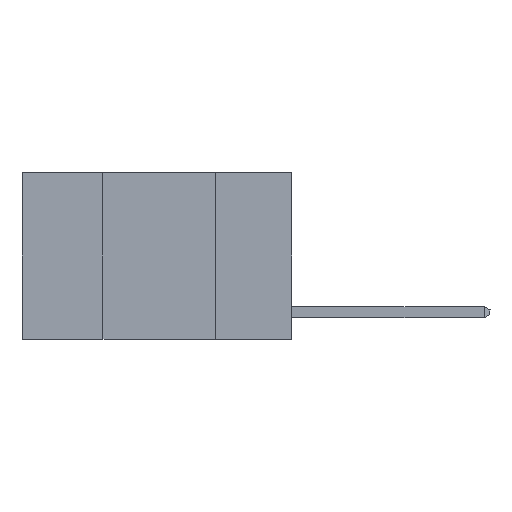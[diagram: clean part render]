
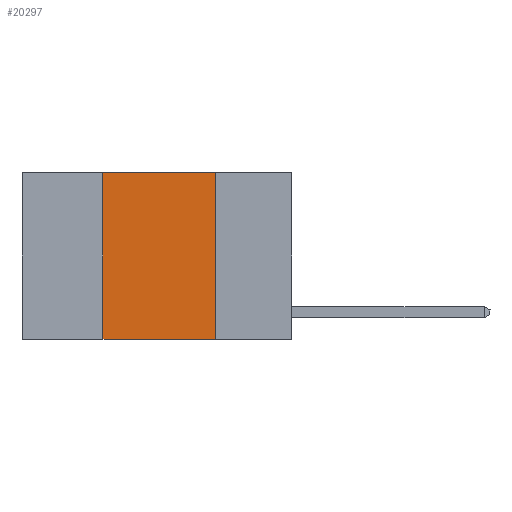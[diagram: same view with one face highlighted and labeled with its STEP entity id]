
A CAD part, left-side view. The second image highlights one B-rep face of the part: STEP entity #20297.
In plain terms, the highlighted planar face has unit normal (-1, 0, 0).
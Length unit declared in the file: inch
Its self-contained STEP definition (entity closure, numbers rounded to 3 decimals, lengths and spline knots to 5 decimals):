
#230 = VERTEX_POINT ( 'NONE', #10636 ) ;
#394 = DIRECTION ( 'NONE',  ( 0., -1., 0. ) ) ;
#1284 = ORIENTED_EDGE ( 'NONE', *, *, #28548, .F. ) ;
#4585 = LINE ( 'NONE', #11406, #22879 ) ;
#5337 = EDGE_CURVE ( 'NONE', #27834, #230, #9714, .T. ) ;
#9714 = LINE ( 'NONE', #11836, #29924 ) ;
#10095 = DIRECTION ( 'NONE',  ( 0., 0., -1. ) ) ;
#10636 = CARTESIAN_POINT ( 'NONE',  ( 0., 0.17, -0.37 ) ) ;
#11406 = CARTESIAN_POINT ( 'NONE',  ( 0., 0.42, 0. ) ) ;
#11836 = CARTESIAN_POINT ( 'NONE',  ( 0., 0.17, 0. ) ) ;
#11877 = CARTESIAN_POINT ( 'NONE',  ( 0., 0.17, 0. ) ) ;
#13815 = DIRECTION ( 'NONE',  ( 0., 0., -1. ) ) ;
#14064 = CARTESIAN_POINT ( 'NONE',  ( 0., 0.6, -0.37 ) ) ;
#15470 = AXIS2_PLACEMENT_3D ( 'NONE', #17219, #26232, #10095 ) ;
#17023 = ORIENTED_EDGE ( 'NONE', *, *, #5337, .F. ) ;
#17112 = ORIENTED_EDGE ( 'NONE', *, *, #17234, .T. ) ;
#17219 = CARTESIAN_POINT ( 'NONE',  ( 0., 0.6, 0. ) ) ;
#17224 = CARTESIAN_POINT ( 'NONE',  ( 0., 0.42, -0.37 ) ) ;
#17234 = EDGE_CURVE ( 'NONE', #21614, #230, #25637, .T. ) ;
#20297 = ADVANCED_FACE ( 'NONE', ( #23789 ), #28659, .F. ) ;
#20781 = VECTOR ( 'NONE', #394, 39.37008 ) ;
#21614 = VERTEX_POINT ( 'NONE', #17224 ) ;
#22252 = EDGE_CURVE ( 'NONE', #21614, #23963, #4585, .T. ) ;
#22475 = LINE ( 'NONE', #25357, #27210 ) ;
#22777 = DIRECTION ( 'NONE',  ( 0., -1., 0. ) ) ;
#22879 = VECTOR ( 'NONE', #25560, 39.37008 ) ;
#23789 = FACE_OUTER_BOUND ( 'NONE', #26074, .T. ) ;
#23963 = VERTEX_POINT ( 'NONE', #28694 ) ;
#25357 = CARTESIAN_POINT ( 'NONE',  ( 0., 0.6, 0. ) ) ;
#25560 = DIRECTION ( 'NONE',  ( 0., 0., 1. ) ) ;
#25637 = LINE ( 'NONE', #14064, #20781 ) ;
#26074 = EDGE_LOOP ( 'NONE', ( #17023, #1284, #29404, #17112 ) ) ;
#26232 = DIRECTION ( 'NONE',  ( 1., 0., 0. ) ) ;
#27210 = VECTOR ( 'NONE', #22777, 39.37008 ) ;
#27834 = VERTEX_POINT ( 'NONE', #11877 ) ;
#28548 = EDGE_CURVE ( 'NONE', #23963, #27834, #22475, .T. ) ;
#28659 = PLANE ( 'NONE',  #15470 ) ;
#28694 = CARTESIAN_POINT ( 'NONE',  ( 0., 0.42, 0. ) ) ;
#29404 = ORIENTED_EDGE ( 'NONE', *, *, #22252, .F. ) ;
#29924 = VECTOR ( 'NONE', #13815, 39.37008 ) ;
